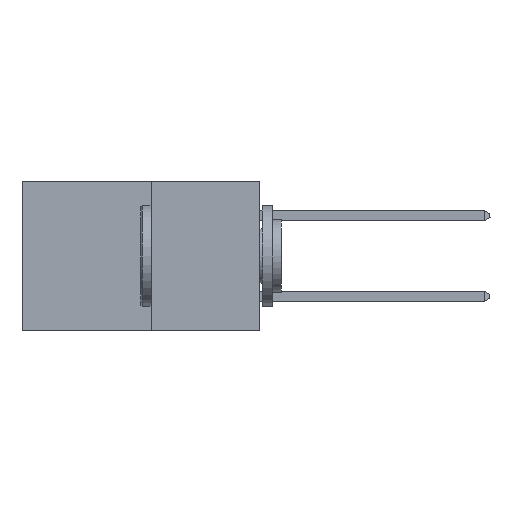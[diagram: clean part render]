
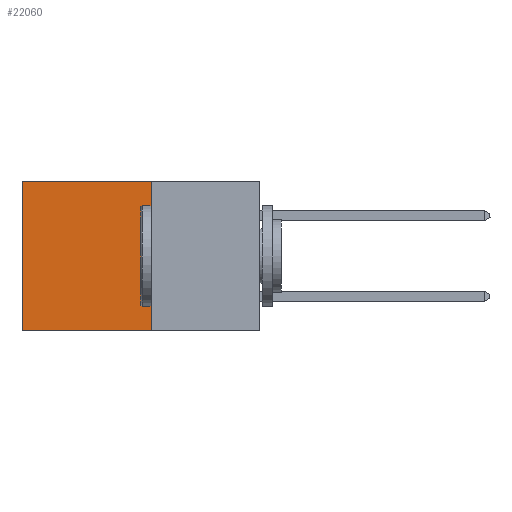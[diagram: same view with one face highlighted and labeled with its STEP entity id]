
A CAD part, left-side view. The second image highlights one B-rep face of the part: STEP entity #22060.
In plain terms, the highlighted planar face has unit normal (-1, 0, 0).
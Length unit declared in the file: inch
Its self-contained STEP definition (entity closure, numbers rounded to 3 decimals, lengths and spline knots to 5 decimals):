
#1650 = ORIENTED_EDGE ( 'NONE', *, *, #15338, .T. ) ;
#2102 = VERTEX_POINT ( 'NONE', #19140 ) ;
#2202 = DIRECTION ( 'NONE',  ( 0., 1., 0. ) ) ;
#2784 = LINE ( 'NONE', #28817, #15828 ) ;
#3059 = LINE ( 'NONE', #16398, #22153 ) ;
#3488 = CARTESIAN_POINT ( 'NONE',  ( 0.277, 0.27, -0.37 ) ) ;
#3987 = EDGE_LOOP ( 'NONE', ( #7692, #5142, #25360, #1650 ) ) ;
#4187 = EDGE_CURVE ( 'NONE', #27969, #2102, #3059, .T. ) ;
#5142 = ORIENTED_EDGE ( 'NONE', *, *, #16401, .F. ) ;
#6624 = CARTESIAN_POINT ( 'NONE',  ( 0.277, 0.27, 0. ) ) ;
#7692 = ORIENTED_EDGE ( 'NONE', *, *, #4187, .T. ) ;
#10072 = AXIS2_PLACEMENT_3D ( 'NONE', #3488, #31994, #26896 ) ;
#11808 = VERTEX_POINT ( 'NONE', #25085 ) ;
#14693 = LINE ( 'NONE', #15222, #26877 ) ;
#15222 = CARTESIAN_POINT ( 'NONE',  ( 0.277, 0.27, 0. ) ) ;
#15338 = EDGE_CURVE ( 'NONE', #33633, #27969, #14693, .T. ) ;
#15699 = EDGE_CURVE ( 'NONE', #33633, #11808, #30100, .T. ) ;
#15828 = VECTOR ( 'NONE', #18458, 39.37008 ) ;
#16398 = CARTESIAN_POINT ( 'NONE',  ( 0.277, 0.59, -0.37 ) ) ;
#16401 = EDGE_CURVE ( 'NONE', #11808, #2102, #2784, .T. ) ;
#16465 = DIRECTION ( 'NONE',  ( 0., 0., -1. ) ) ;
#18458 = DIRECTION ( 'NONE',  ( 0., 1., 0. ) ) ;
#19140 = CARTESIAN_POINT ( 'NONE',  ( 0.277, 0.59, -0.37 ) ) ;
#20764 = CARTESIAN_POINT ( 'NONE',  ( 0.277, 0.59, 0. ) ) ;
#22060 = ADVANCED_FACE ( 'NONE', ( #33251 ), #24268, .F. ) ;
#22153 = VECTOR ( 'NONE', #16465, 39.37008 ) ;
#24268 = PLANE ( 'NONE',  #10072 ) ;
#25085 = CARTESIAN_POINT ( 'NONE',  ( 0.277, 0.27, -0.37 ) ) ;
#25360 = ORIENTED_EDGE ( 'NONE', *, *, #15699, .F. ) ;
#26877 = VECTOR ( 'NONE', #2202, 39.37008 ) ;
#26896 = DIRECTION ( 'NONE',  ( 0., 0., -1. ) ) ;
#27969 = VERTEX_POINT ( 'NONE', #20764 ) ;
#28817 = CARTESIAN_POINT ( 'NONE',  ( 0.277, 0.27, -0.37 ) ) ;
#28966 = CARTESIAN_POINT ( 'NONE',  ( 0.277, 0.27, -0.37 ) ) ;
#29298 = VECTOR ( 'NONE', #31570, 39.37008 ) ;
#30100 = LINE ( 'NONE', #28966, #29298 ) ;
#31570 = DIRECTION ( 'NONE',  ( 0., 0., -1. ) ) ;
#31994 = DIRECTION ( 'NONE',  ( 1., 0., 0. ) ) ;
#33251 = FACE_OUTER_BOUND ( 'NONE', #3987, .T. ) ;
#33633 = VERTEX_POINT ( 'NONE', #6624 ) ;
